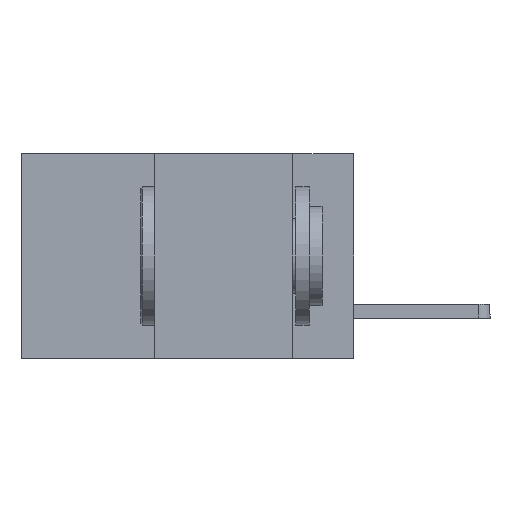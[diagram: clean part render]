
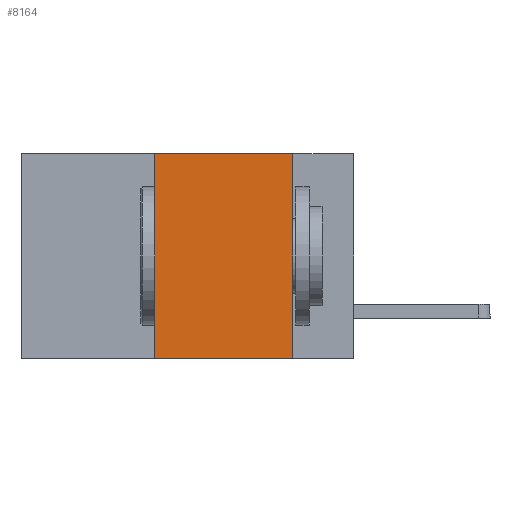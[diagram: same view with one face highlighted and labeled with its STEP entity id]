
A CAD part, left-side view. The second image highlights one B-rep face of the part: STEP entity #8164.
In plain terms, the highlighted planar face has unit normal (-1, 0, 0).
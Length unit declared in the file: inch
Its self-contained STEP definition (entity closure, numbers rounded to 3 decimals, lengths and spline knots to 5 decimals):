
#327 = ORIENTED_EDGE ( 'NONE', *, *, #9588, .F. ) ;
#1224 = CARTESIAN_POINT ( 'NONE',  ( 0., 0.36, -0.37 ) ) ;
#1479 = VERTEX_POINT ( 'NONE', #1224 ) ;
#1591 = LINE ( 'NONE', #9900, #12032 ) ;
#1792 = CARTESIAN_POINT ( 'NONE',  ( 0., 0.6, 0. ) ) ;
#1808 = DIRECTION ( 'NONE',  ( 0., 0., -1. ) ) ;
#3147 = CARTESIAN_POINT ( 'NONE',  ( 0., 0.36, 0. ) ) ;
#3166 = EDGE_CURVE ( 'NONE', #6631, #9220, #8099, .T. ) ;
#3554 = ORIENTED_EDGE ( 'NONE', *, *, #3166, .F. ) ;
#3596 = LINE ( 'NONE', #1792, #5694 ) ;
#3843 = ORIENTED_EDGE ( 'NONE', *, *, #8157, .F. ) ;
#3856 = AXIS2_PLACEMENT_3D ( 'NONE', #6961, #7935, #1808 ) ;
#4387 = CARTESIAN_POINT ( 'NONE',  ( 0., 0.11, -0.37 ) ) ;
#4408 = FACE_OUTER_BOUND ( 'NONE', #9931, .T. ) ;
#4626 = CARTESIAN_POINT ( 'NONE',  ( 0., 0.11, 0. ) ) ;
#4960 = PLANE ( 'NONE',  #3856 ) ;
#5173 = VECTOR ( 'NONE', #8275, 39.37008 ) ;
#5694 = VECTOR ( 'NONE', #8929, 39.37008 ) ;
#6631 = VERTEX_POINT ( 'NONE', #12251 ) ;
#6926 = CARTESIAN_POINT ( 'NONE',  ( 0., 0.6, -0.37 ) ) ;
#6945 = ORIENTED_EDGE ( 'NONE', *, *, #12369, .T. ) ;
#6961 = CARTESIAN_POINT ( 'NONE',  ( 0., 0.6, 0. ) ) ;
#7935 = DIRECTION ( 'NONE',  ( 1., 0., 0. ) ) ;
#8099 = LINE ( 'NONE', #4626, #5173 ) ;
#8157 = EDGE_CURVE ( 'NONE', #1479, #11903, #1591, .T. ) ;
#8164 = ADVANCED_FACE ( 'NONE', ( #4408 ), #4960, .F. ) ;
#8275 = DIRECTION ( 'NONE',  ( 0., 0., -1. ) ) ;
#8929 = DIRECTION ( 'NONE',  ( 0., -1., 0. ) ) ;
#9220 = VERTEX_POINT ( 'NONE', #4387 ) ;
#9428 = LINE ( 'NONE', #6926, #12054 ) ;
#9588 = EDGE_CURVE ( 'NONE', #11903, #6631, #3596, .T. ) ;
#9900 = CARTESIAN_POINT ( 'NONE',  ( 0., 0.36, 0. ) ) ;
#9931 = EDGE_LOOP ( 'NONE', ( #3554, #327, #3843, #6945 ) ) ;
#11903 = VERTEX_POINT ( 'NONE', #3147 ) ;
#12032 = VECTOR ( 'NONE', #12841, 39.37008 ) ;
#12054 = VECTOR ( 'NONE', #12816, 39.37008 ) ;
#12251 = CARTESIAN_POINT ( 'NONE',  ( 0., 0.11, 0. ) ) ;
#12369 = EDGE_CURVE ( 'NONE', #1479, #9220, #9428, .T. ) ;
#12816 = DIRECTION ( 'NONE',  ( 0., -1., 0. ) ) ;
#12841 = DIRECTION ( 'NONE',  ( 0., 0., 1. ) ) ;
